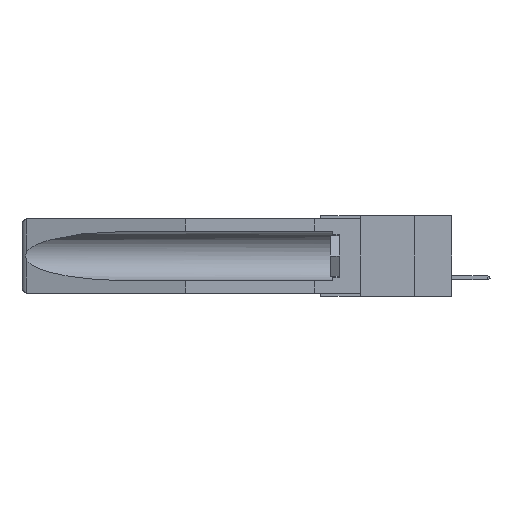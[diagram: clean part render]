
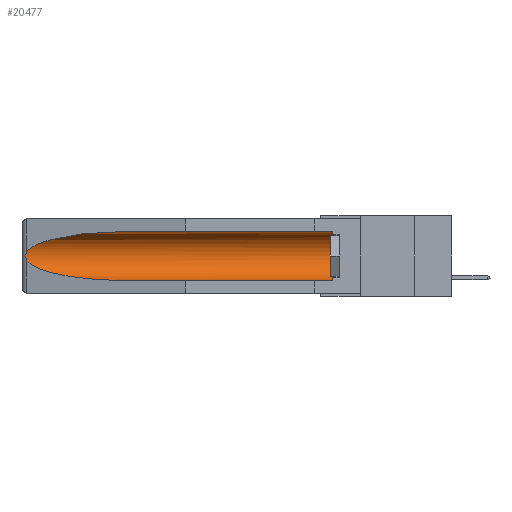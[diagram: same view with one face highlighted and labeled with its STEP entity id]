
A CAD part, left-side view. The second image highlights one B-rep face of the part: STEP entity #20477.
In plain terms, the highlighted cylindrical face has radius 2.857 mm (diameter 5.715 mm), a partial arc.
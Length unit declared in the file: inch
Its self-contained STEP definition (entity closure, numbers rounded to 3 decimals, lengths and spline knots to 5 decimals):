
#373 = B_SPLINE_CURVE_WITH_KNOTS ( 'NONE', 3,
 ( #28347, #30778, #15893, #3740, #18452, #20909, #23324, #8770, #16413, #9475 ),
 .UNSPECIFIED., .F., .F.,
 ( 4, 2, 2, 2, 4 ),
 ( 0., 0.00029, 0.00058, 0.00087, 0.00117 ),
 .UNSPECIFIED. ) ;
#902 = CYLINDRICAL_SURFACE ( 'NONE', #30995, 0.1125 ) ;
#2117 =( BOUNDED_CURVE ( )  B_SPLINE_CURVE ( 3, ( #23494, #23587, #18827, #3805 ),
 .UNSPECIFIED., .F., .F. ) 
 B_SPLINE_CURVE_WITH_KNOTS ( ( 4, 4 ),
 ( 0.1948, 1.5708 ),
 .UNSPECIFIED. ) 
 CURVE ( )  GEOMETRIC_REPRESENTATION_ITEM ( )  RATIONAL_B_SPLINE_CURVE ( ( 1., 0.848, 0.848, 1. ) ) 
 REPRESENTATION_ITEM ( '' )  );
#2562 = ORIENTED_EDGE ( 'NONE', *, *, #8417, .T. ) ;
#3740 = CARTESIAN_POINT ( 'NONE',  ( 0.2673, 1.5327, -0.16383 ) ) ;
#3805 = CARTESIAN_POINT ( 'NONE',  ( 0.155, 1.07973, -0.284 ) ) ;
#3950 = EDGE_CURVE ( 'NONE', #8865, #26567, #26241, .T. ) ;
#4221 = VECTOR ( 'NONE', #8508, 39.37008 ) ;
#4380 = CARTESIAN_POINT ( 'NONE',  ( 0.155, -0.30754, -0.059 ) ) ;
#5121 = ORIENTED_EDGE ( 'NONE', *, *, #30192, .T. ) ;
#5293 = DIRECTION ( 'NONE',  ( 0., -1., 0. ) ) ;
#5560 = AXIS2_PLACEMENT_3D ( 'NONE', #12536, #5293, #24754 ) ;
#6248 = VERTEX_POINT ( 'NONE', #12363 ) ;
#6602 = FACE_OUTER_BOUND ( 'NONE', #12845, .T. ) ;
#7399 = CIRCLE ( 'NONE', #5560, 0.1125 ) ;
#7413 = ORIENTED_EDGE ( 'NONE', *, *, #14605, .T. ) ;
#7542 = DIRECTION ( 'NONE',  ( 0., 1., 0. ) ) ;
#7873 = CARTESIAN_POINT ( 'NONE',  ( 0.26537, 1.52718, -0.14972 ) ) ;
#8417 = EDGE_CURVE ( 'NONE', #22940, #26567, #2117, .T. ) ;
#8508 = DIRECTION ( 'NONE',  ( 0., 1., 0. ) ) ;
#8770 = CARTESIAN_POINT ( 'NONE',  ( 0.26655, 1.53094, -0.18657 ) ) ;
#8865 = VERTEX_POINT ( 'NONE', #15092 ) ;
#8868 = ORIENTED_EDGE ( 'NONE', *, *, #20053, .T. ) ;
#9475 = CARTESIAN_POINT ( 'NONE',  ( 0.26537, 1.52718, -0.19328 ) ) ;
#10820 = CARTESIAN_POINT ( 'NONE',  ( 0.155, -0.30754, -0.284 ) ) ;
#10933 = LINE ( 'NONE', #4380, #17404 ) ;
#12363 = CARTESIAN_POINT ( 'NONE',  ( 0.155, 0.126, -0.059 ) ) ;
#12536 = CARTESIAN_POINT ( 'NONE',  ( 0.155, 0.126, -0.1715 ) ) ;
#12845 = EDGE_LOOP ( 'NONE', ( #8868, #7413, #2562, #16523, #5121, #25727 ) ) ;
#13048 = CARTESIAN_POINT ( 'NONE',  ( 0.25451, 1.48313, -0.09465 ) ) ;
#14015 =( BOUNDED_CURVE ( )  B_SPLINE_CURVE ( 3, ( #29892, #30000, #13048, #24732 ),
 .UNSPECIFIED., .F., .T. ) 
 B_SPLINE_CURVE_WITH_KNOTS ( ( 4, 4 ),
 ( 4.71239, 6.08839 ),
 .UNSPECIFIED. ) 
 CURVE ( )  GEOMETRIC_REPRESENTATION_ITEM ( )  RATIONAL_B_SPLINE_CURVE ( ( 1., 0.848, 0.848, 1. ) ) 
 REPRESENTATION_ITEM ( '' )  );
#14605 = EDGE_CURVE ( 'NONE', #26797, #22940, #373, .T. ) ;
#15092 = CARTESIAN_POINT ( 'NONE',  ( 0.155, 0.126, -0.284 ) ) ;
#15893 = CARTESIAN_POINT ( 'NONE',  ( 0.26654, 1.53092, -0.15636 ) ) ;
#15903 = CARTESIAN_POINT ( 'NONE',  ( 0.155, -0.30754, -0.1715 ) ) ;
#16413 = CARTESIAN_POINT ( 'NONE',  ( 0.26597, 1.5296, -0.19026 ) ) ;
#16523 = ORIENTED_EDGE ( 'NONE', *, *, #3950, .F. ) ;
#17035 = CARTESIAN_POINT ( 'NONE',  ( 0.155, 1.07973, -0.059 ) ) ;
#17404 = VECTOR ( 'NONE', #7542, 39.37008 ) ;
#18358 = DIRECTION ( 'NONE',  ( 0., 0., 1. ) ) ;
#18452 = CARTESIAN_POINT ( 'NONE',  ( 0.2675, 1.53308, -0.16763 ) ) ;
#18772 = EDGE_CURVE ( 'NONE', #6248, #18774, #10933, .T. ) ;
#18774 = VERTEX_POINT ( 'NONE', #17035 ) ;
#18827 = CARTESIAN_POINT ( 'NONE',  ( 0.21114, 1.30732, -0.284 ) ) ;
#20053 = EDGE_CURVE ( 'NONE', #18774, #26797, #14015, .T. ) ;
#20477 = ADVANCED_FACE ( 'NONE', ( #6602 ), #902, .F. ) ;
#20709 = DIRECTION ( 'NONE',  ( 0., 1., 0. ) ) ;
#20909 = CARTESIAN_POINT ( 'NONE',  ( 0.2675, 1.53308, -0.17534 ) ) ;
#22940 = VERTEX_POINT ( 'NONE', #29084 ) ;
#23324 = CARTESIAN_POINT ( 'NONE',  ( 0.2673, 1.53269, -0.17917 ) ) ;
#23494 = CARTESIAN_POINT ( 'NONE',  ( 0.26537, 1.52718, -0.19328 ) ) ;
#23587 = CARTESIAN_POINT ( 'NONE',  ( 0.25451, 1.48313, -0.24835 ) ) ;
#24732 = CARTESIAN_POINT ( 'NONE',  ( 0.26537, 1.52718, -0.14972 ) ) ;
#24754 = DIRECTION ( 'NONE',  ( 0., 0., 1. ) ) ;
#25727 = ORIENTED_EDGE ( 'NONE', *, *, #18772, .T. ) ;
#26241 = LINE ( 'NONE', #10820, #4221 ) ;
#26567 = VERTEX_POINT ( 'NONE', #30870 ) ;
#26797 = VERTEX_POINT ( 'NONE', #7873 ) ;
#28347 = CARTESIAN_POINT ( 'NONE',  ( 0.26537, 1.52718, -0.14972 ) ) ;
#29084 = CARTESIAN_POINT ( 'NONE',  ( 0.26537, 1.52718, -0.19328 ) ) ;
#29892 = CARTESIAN_POINT ( 'NONE',  ( 0.155, 1.07973, -0.059 ) ) ;
#30000 = CARTESIAN_POINT ( 'NONE',  ( 0.21114, 1.30732, -0.059 ) ) ;
#30192 = EDGE_CURVE ( 'NONE', #8865, #6248, #7399, .T. ) ;
#30778 = CARTESIAN_POINT ( 'NONE',  ( 0.26597, 1.52961, -0.15275 ) ) ;
#30870 = CARTESIAN_POINT ( 'NONE',  ( 0.155, 1.07973, -0.284 ) ) ;
#30995 = AXIS2_PLACEMENT_3D ( 'NONE', #15903, #20709, #18358 ) ;
